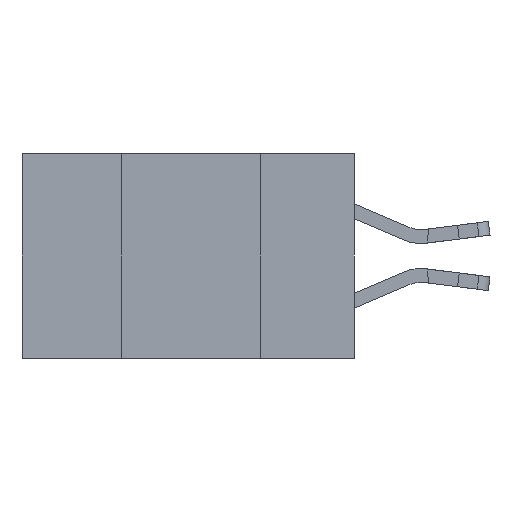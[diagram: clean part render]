
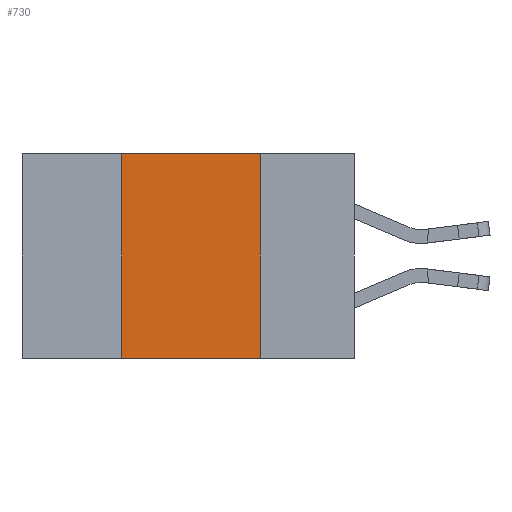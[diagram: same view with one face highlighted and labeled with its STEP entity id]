
A CAD part, left-side view. The second image highlights one B-rep face of the part: STEP entity #730.
In plain terms, the highlighted planar face has unit normal (-1, 0, 0).
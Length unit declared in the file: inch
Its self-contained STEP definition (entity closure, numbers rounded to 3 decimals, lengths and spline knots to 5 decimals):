
#132 = EDGE_CURVE ( 'NONE', #22178, #17004, #24482, .T. ) ;
#730 = ADVANCED_FACE ( 'NONE', ( #25127 ), #15469, .F. ) ;
#1176 = CARTESIAN_POINT ( 'NONE',  ( 0., 0.17, -0.37 ) ) ;
#1644 = CARTESIAN_POINT ( 'NONE',  ( 0., 0.42, 0. ) ) ;
#2041 = ORIENTED_EDGE ( 'NONE', *, *, #8820, .F. ) ;
#2127 = LINE ( 'NONE', #9708, #8141 ) ;
#3141 = VECTOR ( 'NONE', #4298, 39.37008 ) ;
#3650 = DIRECTION ( 'NONE',  ( 0., 0., 1. ) ) ;
#4298 = DIRECTION ( 'NONE',  ( 0., -1., 0. ) ) ;
#5019 = CARTESIAN_POINT ( 'NONE',  ( 0., 0.42, 0. ) ) ;
#6224 = EDGE_CURVE ( 'NONE', #17004, #17106, #18677, .T. ) ;
#8141 = VECTOR ( 'NONE', #23683, 39.37008 ) ;
#8777 = CARTESIAN_POINT ( 'NONE',  ( 0., 0.17, 0. ) ) ;
#8820 = EDGE_CURVE ( 'NONE', #19186, #22178, #13366, .T. ) ;
#9708 = CARTESIAN_POINT ( 'NONE',  ( 0., 0.6, -0.37 ) ) ;
#11098 = CARTESIAN_POINT ( 'NONE',  ( 0., 0.42, -0.37 ) ) ;
#11715 = CARTESIAN_POINT ( 'NONE',  ( 0., 0.17, 0. ) ) ;
#11728 = CARTESIAN_POINT ( 'NONE',  ( 0., 0.6, 0. ) ) ;
#13366 = LINE ( 'NONE', #1644, #23952 ) ;
#14011 = VECTOR ( 'NONE', #17747, 39.37008 ) ;
#14605 = DIRECTION ( 'NONE',  ( 0., 0., -1. ) ) ;
#14634 = DIRECTION ( 'NONE',  ( 1., 0., 0. ) ) ;
#14790 = CARTESIAN_POINT ( 'NONE',  ( 0., 0.6, 0. ) ) ;
#15469 = PLANE ( 'NONE',  #19422 ) ;
#17004 = VERTEX_POINT ( 'NONE', #8777 ) ;
#17106 = VERTEX_POINT ( 'NONE', #1176 ) ;
#17747 = DIRECTION ( 'NONE',  ( 0., 0., -1. ) ) ;
#18677 = LINE ( 'NONE', #11715, #14011 ) ;
#19026 = ORIENTED_EDGE ( 'NONE', *, *, #132, .F. ) ;
#19186 = VERTEX_POINT ( 'NONE', #11098 ) ;
#19346 = EDGE_CURVE ( 'NONE', #19186, #17106, #2127, .T. ) ;
#19422 = AXIS2_PLACEMENT_3D ( 'NONE', #11728, #14634, #14605 ) ;
#20026 = ORIENTED_EDGE ( 'NONE', *, *, #19346, .T. ) ;
#22178 = VERTEX_POINT ( 'NONE', #5019 ) ;
#23683 = DIRECTION ( 'NONE',  ( 0., -1., 0. ) ) ;
#23952 = VECTOR ( 'NONE', #3650, 39.37008 ) ;
#24482 = LINE ( 'NONE', #14790, #3141 ) ;
#25127 = FACE_OUTER_BOUND ( 'NONE', #25776, .T. ) ;
#25212 = ORIENTED_EDGE ( 'NONE', *, *, #6224, .F. ) ;
#25776 = EDGE_LOOP ( 'NONE', ( #25212, #19026, #2041, #20026 ) ) ;
